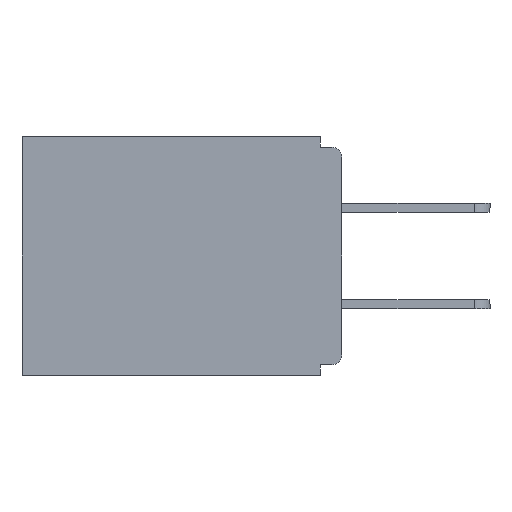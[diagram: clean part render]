
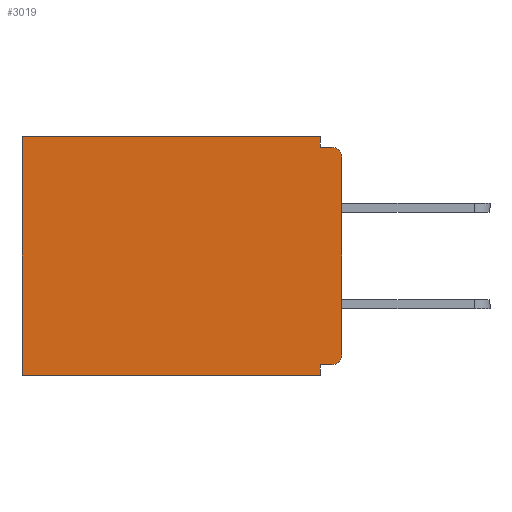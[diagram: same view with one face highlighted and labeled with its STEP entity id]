
A CAD part, left-side view. The second image highlights one B-rep face of the part: STEP entity #3019.
In plain terms, the highlighted planar face has unit normal (-1, 0, 0).
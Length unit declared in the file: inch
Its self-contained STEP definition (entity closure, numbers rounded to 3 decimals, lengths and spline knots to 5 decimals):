
#314 = CARTESIAN_POINT ( 'NONE',  ( 0.298, 0.031, 0. ) ) ;
#652 = DIRECTION ( 'NONE',  ( 0., 0., -1. ) ) ;
#1254 = AXIS2_PLACEMENT_3D ( 'NONE', #8238, #9317, #14000 ) ;
#1348 = CARTESIAN_POINT ( 'NONE',  ( 0.298, 0.031, -0.328 ) ) ;
#1372 = VERTEX_POINT ( 'NONE', #6210 ) ;
#1619 = DIRECTION ( 'NONE',  ( 0., 0., -1. ) ) ;
#1690 = ORIENTED_EDGE ( 'NONE', *, *, #5101, .F. ) ;
#1734 = CARTESIAN_POINT ( 'NONE',  ( 0.298, 0., 0. ) ) ;
#1838 = CIRCLE ( 'NONE', #13141, 0.015 ) ;
#2012 = CARTESIAN_POINT ( 'NONE',  ( 0.298, 0.015, -0.015 ) ) ;
#2272 = LINE ( 'NONE', #4526, #11350 ) ;
#2340 = DIRECTION ( 'NONE',  ( 0., 0., -1. ) ) ;
#2368 = VECTOR ( 'NONE', #4646, 39.37008 ) ;
#2507 = ORIENTED_EDGE ( 'NONE', *, *, #4627, .T. ) ;
#2703 = CARTESIAN_POINT ( 'NONE',  ( 0.298, 0.46, -0.343 ) ) ;
#2749 = LINE ( 'NONE', #1734, #2368 ) ;
#2881 = ORIENTED_EDGE ( 'NONE', *, *, #5442, .F. ) ;
#2912 = LINE ( 'NONE', #3790, #15076 ) ;
#2949 = EDGE_CURVE ( 'NONE', #10794, #14963, #2749, .T. ) ;
#3019 = ADVANCED_FACE ( 'NONE', ( #6251 ), #7474, .F. ) ;
#3125 = VECTOR ( 'NONE', #652, 39.37008 ) ;
#3511 = CARTESIAN_POINT ( 'NONE',  ( 0.298, 0., 0. ) ) ;
#3608 = CARTESIAN_POINT ( 'NONE',  ( 0.298, 0.015, -0.03 ) ) ;
#3652 = LINE ( 'NONE', #7674, #3125 ) ;
#3742 = CIRCLE ( 'NONE', #1254, 0.015 ) ;
#3772 = VERTEX_POINT ( 'NONE', #6813 ) ;
#3790 = CARTESIAN_POINT ( 'NONE',  ( 0.298, 0., -0.328 ) ) ;
#3914 = CARTESIAN_POINT ( 'NONE',  ( 0.298, 0.031, -0.343 ) ) ;
#4337 = ORIENTED_EDGE ( 'NONE', *, *, #11349, .F. ) ;
#4525 = ORIENTED_EDGE ( 'NONE', *, *, #9079, .T. ) ;
#4526 = CARTESIAN_POINT ( 'NONE',  ( 0.298, 0., -0.343 ) ) ;
#4627 = EDGE_CURVE ( 'NONE', #3772, #11165, #1838, .T. ) ;
#4646 = DIRECTION ( 'NONE',  ( 0., 1., 0. ) ) ;
#4693 = EDGE_LOOP ( 'NONE', ( #2507, #9643, #1690, #9486, #4525, #12905, #13476, #2881, #10256, #4337 ) ) ;
#4974 = VECTOR ( 'NONE', #9434, 39.37008 ) ;
#5036 = CARTESIAN_POINT ( 'NONE',  ( 0.298, 0.015, -0.328 ) ) ;
#5059 = LINE ( 'NONE', #7032, #8587 ) ;
#5101 = EDGE_CURVE ( 'NONE', #10794, #15008, #10328, .T. ) ;
#5115 = CARTESIAN_POINT ( 'NONE',  ( 0.298, 0., 0. ) ) ;
#5295 = EDGE_CURVE ( 'NONE', #6618, #1372, #3652, .T. ) ;
#5442 = EDGE_CURVE ( 'NONE', #11417, #6618, #2912, .T. ) ;
#5449 = CARTESIAN_POINT ( 'NONE',  ( 0.298, 0.031, -0.015 ) ) ;
#5677 = DIRECTION ( 'NONE',  ( 0., -1., 0. ) ) ;
#5997 = CARTESIAN_POINT ( 'NONE',  ( 0.298, 0.46, 0. ) ) ;
#6210 = CARTESIAN_POINT ( 'NONE',  ( 0.298, 0.031, -0.343 ) ) ;
#6251 = FACE_OUTER_BOUND ( 'NONE', #4693, .T. ) ;
#6618 = VERTEX_POINT ( 'NONE', #1348 ) ;
#6813 = CARTESIAN_POINT ( 'NONE',  ( 0.298, 0., -0.03 ) ) ;
#6919 = CARTESIAN_POINT ( 'NONE',  ( 0.298, 0.46, 0. ) ) ;
#7001 = VERTEX_POINT ( 'NONE', #12359 ) ;
#7032 = CARTESIAN_POINT ( 'NONE',  ( 0.298, 0., -0.015 ) ) ;
#7429 = DIRECTION ( 'NONE',  ( 0., 1., 0. ) ) ;
#7474 = PLANE ( 'NONE',  #14816 ) ;
#7674 = CARTESIAN_POINT ( 'NONE',  ( 0.298, 0.031, -0.343 ) ) ;
#7693 = VERTEX_POINT ( 'NONE', #2703 ) ;
#8238 = CARTESIAN_POINT ( 'NONE',  ( 0.298, 0.015, -0.313 ) ) ;
#8368 = DIRECTION ( 'NONE',  ( -1., 0., 0. ) ) ;
#8587 = VECTOR ( 'NONE', #5677, 39.37008 ) ;
#8591 = DIRECTION ( 'NONE',  ( 1., 0., 0. ) ) ;
#8672 = EDGE_CURVE ( 'NONE', #1372, #7693, #2272, .T. ) ;
#9058 = EDGE_CURVE ( 'NONE', #11417, #7001, #3742, .T. ) ;
#9079 = EDGE_CURVE ( 'NONE', #14963, #7693, #10950, .T. ) ;
#9317 = DIRECTION ( 'NONE',  ( -1., 0., 0. ) ) ;
#9434 = DIRECTION ( 'NONE',  ( 0., 0., -1. ) ) ;
#9486 = ORIENTED_EDGE ( 'NONE', *, *, #2949, .T. ) ;
#9643 = ORIENTED_EDGE ( 'NONE', *, *, #14838, .F. ) ;
#9880 = DIRECTION ( 'NONE',  ( 0., 0., -1. ) ) ;
#10256 = ORIENTED_EDGE ( 'NONE', *, *, #9058, .T. ) ;
#10328 = LINE ( 'NONE', #3914, #13069 ) ;
#10543 = DIRECTION ( 'NONE',  ( 0., 0., -1. ) ) ;
#10794 = VERTEX_POINT ( 'NONE', #314 ) ;
#10950 = LINE ( 'NONE', #6919, #12793 ) ;
#11165 = VERTEX_POINT ( 'NONE', #2012 ) ;
#11349 = EDGE_CURVE ( 'NONE', #3772, #7001, #13281, .T. ) ;
#11350 = VECTOR ( 'NONE', #13178, 39.37008 ) ;
#11417 = VERTEX_POINT ( 'NONE', #5036 ) ;
#12359 = CARTESIAN_POINT ( 'NONE',  ( 0.298, 0., -0.313 ) ) ;
#12793 = VECTOR ( 'NONE', #2340, 39.37008 ) ;
#12905 = ORIENTED_EDGE ( 'NONE', *, *, #8672, .F. ) ;
#13069 = VECTOR ( 'NONE', #9880, 39.37008 ) ;
#13141 = AXIS2_PLACEMENT_3D ( 'NONE', #3608, #8368, #10543 ) ;
#13178 = DIRECTION ( 'NONE',  ( 0., 1., 0. ) ) ;
#13281 = LINE ( 'NONE', #3511, #4974 ) ;
#13476 = ORIENTED_EDGE ( 'NONE', *, *, #5295, .F. ) ;
#14000 = DIRECTION ( 'NONE',  ( 0., 0., -1. ) ) ;
#14816 = AXIS2_PLACEMENT_3D ( 'NONE', #5115, #8591, #1619 ) ;
#14838 = EDGE_CURVE ( 'NONE', #15008, #11165, #5059, .T. ) ;
#14963 = VERTEX_POINT ( 'NONE', #5997 ) ;
#15008 = VERTEX_POINT ( 'NONE', #5449 ) ;
#15076 = VECTOR ( 'NONE', #7429, 39.37008 ) ;
